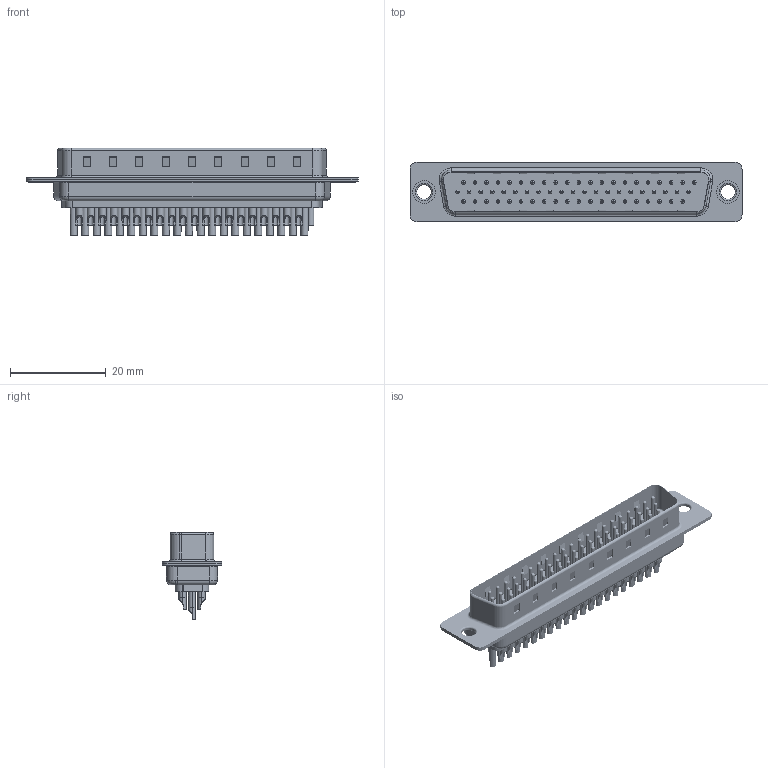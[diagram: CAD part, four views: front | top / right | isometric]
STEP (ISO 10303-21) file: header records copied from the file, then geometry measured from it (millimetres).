
FILE_DESCRIPTION (( 'STEP AP203' ), '1' );
FILE_NAME ('637-M62-332-BT1.STEP', '2018-11-20T02:51:39', ( '' ), ( '' ), 'SwSTEP 2.0', 'SolidWorks 2016', '' );
FILE_SCHEMA (( 'CONFIG_CONTROL_DESIGN' ));
Length unit declared in the file: millimetre
Products named in the file (8): 637M Contact Row 1_32; 637M Contact Row 2_32; 637M Contact Row 3_32; 637M Thru Hole Rivet; 637-M62-332-BT1; 637M Housing_62 Contacts; 637M Shell Front_62 Contacts; 637M Shell Rear_62 Contacts
Assembly tree (67 placements, depth 2):
  637-M62-332-BT1
    637M Housing_62 Contacts
    637M Shell Front_62 Contacts
    637M Shell Rear_62 Contacts
    637M Contact Row 1_32  x21
    637M Contact Row 2_32  x21
    637M Contact Row 3_32  x20
    637M Thru Hole Rivet  x2
Bounding box: 69.4 x 12.5 x 18.25 mm (x, y, z)
Volume: 4044.3 mm3; surface area: 12031.7 mm2
Topology: 67 solids, 67 shells, 2680 faces, 6183 edges, 3772 vertices
Faces by surface type: cylinder 1117, plane 761, torus 678, cone 124
Entity records: 30838 total; most frequent: DIRECTION 5383, CARTESIAN_POINT 4881, ORIENTED_EDGE 4486, EDGE_CURVE 2243, AXIS2_PLACEMENT_3D 2166, VERTEX_POINT 1447, EDGE_LOOP 1262, CIRCLE 1147
